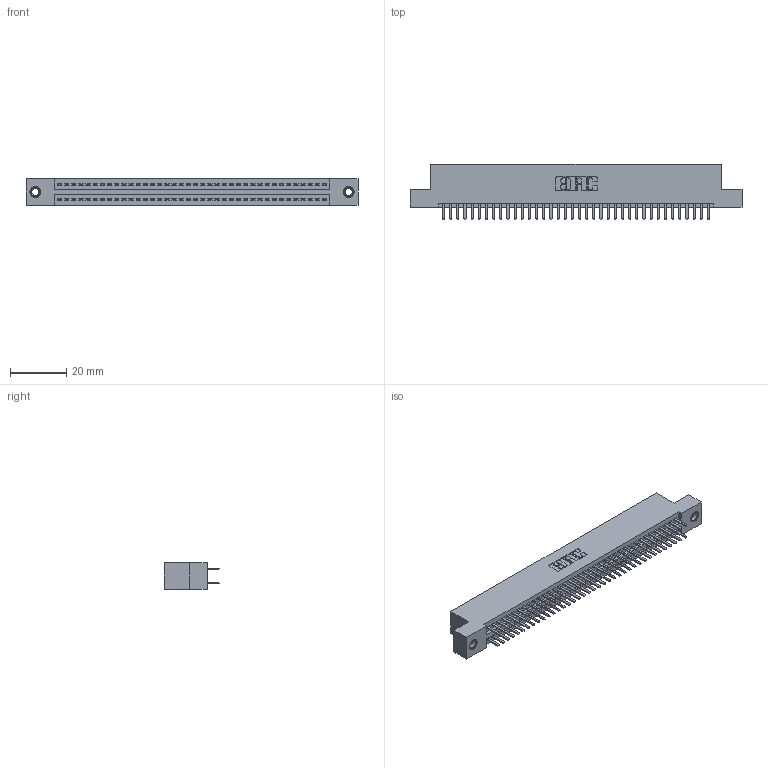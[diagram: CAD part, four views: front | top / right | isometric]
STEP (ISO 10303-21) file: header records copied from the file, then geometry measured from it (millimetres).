
FILE_DESCRIPTION (( 'STEP AP203' ), '1' );
FILE_NAME ('345-076-520-207.STEP', '2018-10-02T14:57:44', ( '' ), ( '' ), 'SwSTEP 2.0', 'SolidWorks 2016', '' );
FILE_SCHEMA (( 'CONFIG_CONTROL_DESIGN' ));
Length unit declared in the file: inch
Products named in the file (4): 345 Part_Flush Mounting Lugs - 0.156 Dia-TI; 345-292-001_345-293-120; 345-076-520-207; 345-250-001_345-250-005-103
Assembly tree (79 placements, depth 2):
  345-076-520-207
    345 Part_Flush Mounting Lugs - 0.156 Dia-TI
    345-292-001_345-293-120  x76
    345-250-001_345-250-005-103  x2
Bounding box: 117.73 x 19.68 x 9.4 mm (x, y, z)
Volume: 11352.3 mm3; surface area: 16659.9 mm2
Topology: 79 solids, 79 shells, 4290 faces, 12409 edges, 8062 vertices
Faces by surface type: plane 2772, cylinder 1502, cone 12, torus 4
Entity records: 31654 total; most frequent: CARTESIAN_POINT 5303, ORIENTED_EDGE 5218, DIRECTION 4695, EDGE_CURVE 2609, VECTOR 2301, LINE 2301, VERTEX_POINT 1732, AXIS2_PLACEMENT_3D 1197
